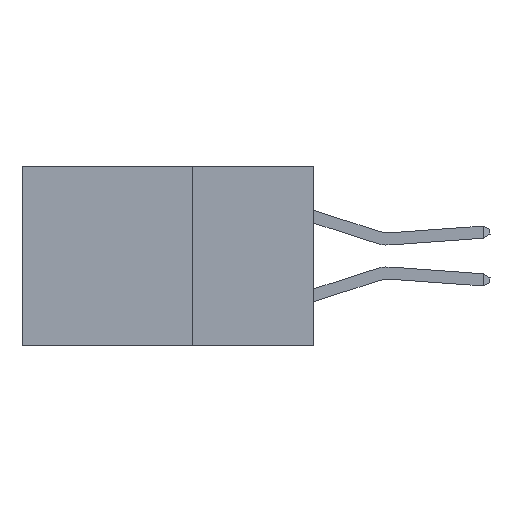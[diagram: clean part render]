
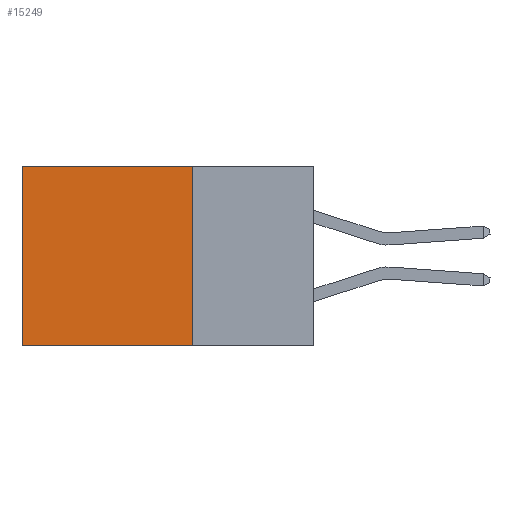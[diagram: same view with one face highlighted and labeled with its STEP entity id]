
A CAD part, left-side view. The second image highlights one B-rep face of the part: STEP entity #15249.
In plain terms, the highlighted planar face has unit normal (-1, 0, 0).
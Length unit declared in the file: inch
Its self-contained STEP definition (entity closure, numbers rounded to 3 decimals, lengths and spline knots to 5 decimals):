
#504 = DIRECTION ( 'NONE',  ( 0., 0., -1. ) ) ;
#576 = VECTOR ( 'NONE', #27237, 39.37008 ) ;
#779 = CARTESIAN_POINT ( 'NONE',  ( 0.2875, 0.25, 0. ) ) ;
#2390 = PLANE ( 'NONE',  #31377 ) ;
#5661 = CARTESIAN_POINT ( 'NONE',  ( 0.2875, 0.25, 0. ) ) ;
#5943 = LINE ( 'NONE', #27532, #7737 ) ;
#7737 = VECTOR ( 'NONE', #30629, 39.37008 ) ;
#8015 = LINE ( 'NONE', #5661, #25549 ) ;
#9596 = CARTESIAN_POINT ( 'NONE',  ( 0.2875, 0.25, -0.37 ) ) ;
#12080 = ORIENTED_EDGE ( 'NONE', *, *, #29261, .F. ) ;
#13516 = DIRECTION ( 'NONE',  ( 0., 0., -1. ) ) ;
#14952 = EDGE_LOOP ( 'NONE', ( #19642, #12080, #15822, #32531 ) ) ;
#15249 = ADVANCED_FACE ( 'NONE', ( #27876 ), #2390, .F. ) ;
#15822 = ORIENTED_EDGE ( 'NONE', *, *, #29090, .F. ) ;
#15979 = EDGE_CURVE ( 'NONE', #20955, #25769, #8015, .T. ) ;
#17272 = LINE ( 'NONE', #9596, #576 ) ;
#18157 = CARTESIAN_POINT ( 'NONE',  ( 0.2875, 0.6, 0. ) ) ;
#18363 = LINE ( 'NONE', #29878, #24817 ) ;
#19642 = ORIENTED_EDGE ( 'NONE', *, *, #28578, .T. ) ;
#19990 = CARTESIAN_POINT ( 'NONE',  ( 0.2875, 0.25, 0. ) ) ;
#20955 = VERTEX_POINT ( 'NONE', #779 ) ;
#22985 = CARTESIAN_POINT ( 'NONE',  ( 0.2875, 0.25, -0.37 ) ) ;
#24817 = VECTOR ( 'NONE', #504, 39.37008 ) ;
#25549 = VECTOR ( 'NONE', #30544, 39.37008 ) ;
#25769 = VERTEX_POINT ( 'NONE', #18157 ) ;
#27237 = DIRECTION ( 'NONE',  ( 0., 1., 0. ) ) ;
#27532 = CARTESIAN_POINT ( 'NONE',  ( 0.2875, 0.25, 0. ) ) ;
#27876 = FACE_OUTER_BOUND ( 'NONE', #14952, .T. ) ;
#28578 = EDGE_CURVE ( 'NONE', #25769, #32161, #18363, .T. ) ;
#29090 = EDGE_CURVE ( 'NONE', #20955, #33066, #5943, .T. ) ;
#29261 = EDGE_CURVE ( 'NONE', #33066, #32161, #17272, .T. ) ;
#29878 = CARTESIAN_POINT ( 'NONE',  ( 0.2875, 0.6, 0. ) ) ;
#30544 = DIRECTION ( 'NONE',  ( 0., 1., 0. ) ) ;
#30629 = DIRECTION ( 'NONE',  ( 0., 0., -1. ) ) ;
#31377 = AXIS2_PLACEMENT_3D ( 'NONE', #19990, #31686, #13516 ) ;
#31686 = DIRECTION ( 'NONE',  ( 1., 0., 0. ) ) ;
#32161 = VERTEX_POINT ( 'NONE', #37015 ) ;
#32531 = ORIENTED_EDGE ( 'NONE', *, *, #15979, .T. ) ;
#33066 = VERTEX_POINT ( 'NONE', #22985 ) ;
#37015 = CARTESIAN_POINT ( 'NONE',  ( 0.2875, 0.6, -0.37 ) ) ;
